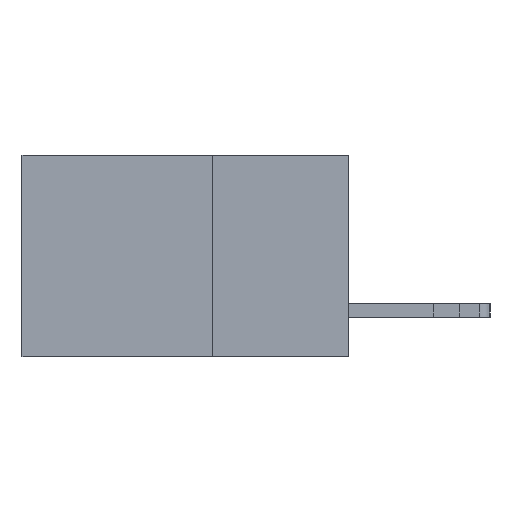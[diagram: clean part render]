
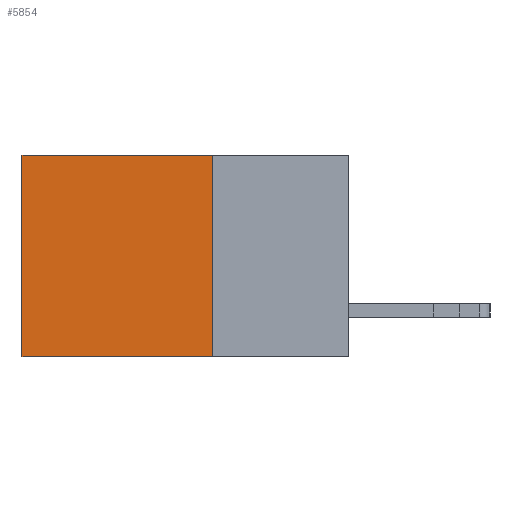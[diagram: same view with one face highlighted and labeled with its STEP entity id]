
A CAD part, left-side view. The second image highlights one B-rep face of the part: STEP entity #5854.
In plain terms, the highlighted planar face has unit normal (-1, 0, 0).
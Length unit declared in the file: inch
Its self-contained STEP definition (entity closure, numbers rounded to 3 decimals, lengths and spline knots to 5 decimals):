
#87 = EDGE_CURVE ( 'NONE', #7169, #6485, #7670, .T. ) ;
#539 = CARTESIAN_POINT ( 'NONE',  ( 0.298, 0.25, -0.37 ) ) ;
#708 = LINE ( 'NONE', #6340, #10360 ) ;
#808 = CARTESIAN_POINT ( 'NONE',  ( 0.298, 0.6, 0. ) ) ;
#1224 = LINE ( 'NONE', #539, #3502 ) ;
#1300 = CARTESIAN_POINT ( 'NONE',  ( 0.298, 0.25, 0. ) ) ;
#1335 = EDGE_CURVE ( 'NONE', #6485, #1516, #3592, .T. ) ;
#1357 = EDGE_CURVE ( 'NONE', #7169, #7528, #708, .T. ) ;
#1516 = VERTEX_POINT ( 'NONE', #2442 ) ;
#2442 = CARTESIAN_POINT ( 'NONE',  ( 0.298, 0.6, -0.37 ) ) ;
#3011 = CARTESIAN_POINT ( 'NONE',  ( 0.298, 0.25, 0. ) ) ;
#3190 = AXIS2_PLACEMENT_3D ( 'NONE', #11527, #11564, #6132 ) ;
#3283 = ORIENTED_EDGE ( 'NONE', *, *, #1335, .T. ) ;
#3309 = PLANE ( 'NONE',  #3190 ) ;
#3502 = VECTOR ( 'NONE', #7202, 39.37008 ) ;
#3556 = CARTESIAN_POINT ( 'NONE',  ( 0.298, 0.25, -0.37 ) ) ;
#3592 = LINE ( 'NONE', #808, #3858 ) ;
#3858 = VECTOR ( 'NONE', #10471, 39.37008 ) ;
#5516 = ORIENTED_EDGE ( 'NONE', *, *, #6211, .F. ) ;
#5854 = ADVANCED_FACE ( 'NONE', ( #10974 ), #3309, .F. ) ;
#6132 = DIRECTION ( 'NONE',  ( 0., 0., -1. ) ) ;
#6211 = EDGE_CURVE ( 'NONE', #7528, #1516, #1224, .T. ) ;
#6340 = CARTESIAN_POINT ( 'NONE',  ( 0.298, 0.25, 0. ) ) ;
#6485 = VERTEX_POINT ( 'NONE', #8456 ) ;
#7169 = VERTEX_POINT ( 'NONE', #3011 ) ;
#7202 = DIRECTION ( 'NONE',  ( 0., 1., 0. ) ) ;
#7528 = VERTEX_POINT ( 'NONE', #3556 ) ;
#7670 = LINE ( 'NONE', #1300, #9836 ) ;
#7699 = DIRECTION ( 'NONE',  ( 0., 1., 0. ) ) ;
#8304 = EDGE_LOOP ( 'NONE', ( #3283, #5516, #8511, #10671 ) ) ;
#8456 = CARTESIAN_POINT ( 'NONE',  ( 0.298, 0.6, 0. ) ) ;
#8511 = ORIENTED_EDGE ( 'NONE', *, *, #1357, .F. ) ;
#9366 = DIRECTION ( 'NONE',  ( 0., 0., -1. ) ) ;
#9836 = VECTOR ( 'NONE', #7699, 39.37008 ) ;
#10360 = VECTOR ( 'NONE', #9366, 39.37008 ) ;
#10471 = DIRECTION ( 'NONE',  ( 0., 0., -1. ) ) ;
#10671 = ORIENTED_EDGE ( 'NONE', *, *, #87, .T. ) ;
#10974 = FACE_OUTER_BOUND ( 'NONE', #8304, .T. ) ;
#11527 = CARTESIAN_POINT ( 'NONE',  ( 0.298, 0.25, 0. ) ) ;
#11564 = DIRECTION ( 'NONE',  ( 1., 0., 0. ) ) ;
